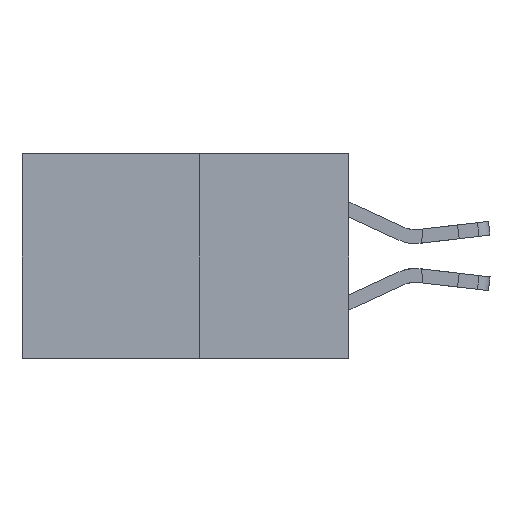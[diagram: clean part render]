
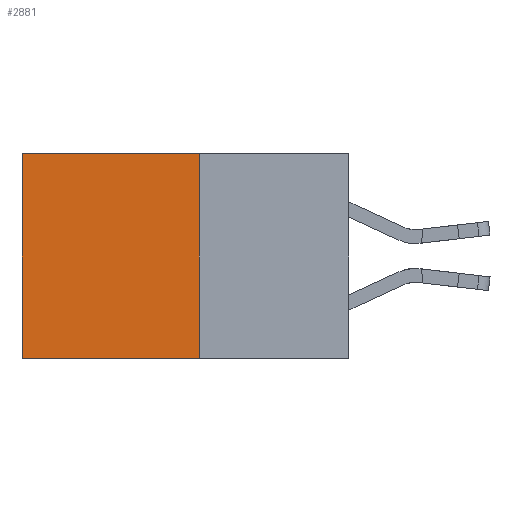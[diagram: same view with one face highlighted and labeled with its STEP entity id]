
A CAD part, left-side view. The second image highlights one B-rep face of the part: STEP entity #2881.
In plain terms, the highlighted planar face has unit normal (-1, 0, 0).
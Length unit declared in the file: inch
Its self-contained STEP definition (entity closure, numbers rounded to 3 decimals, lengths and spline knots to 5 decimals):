
#1489 = EDGE_CURVE ( 'NONE', #11108, #1979, #19267, .T. ) ;
#1666 = CARTESIAN_POINT ( 'NONE',  ( 0.277, 0.59, 0. ) ) ;
#1736 = LINE ( 'NONE', #14465, #20561 ) ;
#1979 = VERTEX_POINT ( 'NONE', #4286 ) ;
#2881 = ADVANCED_FACE ( 'NONE', ( #22049 ), #15849, .F. ) ;
#4286 = CARTESIAN_POINT ( 'NONE',  ( 0.277, 0.27, -0.37 ) ) ;
#4748 = DIRECTION ( 'NONE',  ( 1., 0., 0. ) ) ;
#5076 = VECTOR ( 'NONE', #12967, 39.37008 ) ;
#5095 = DIRECTION ( 'NONE',  ( 0., 1., 0. ) ) ;
#5452 = CARTESIAN_POINT ( 'NONE',  ( 0.277, 0.27, 0. ) ) ;
#7298 = ORIENTED_EDGE ( 'NONE', *, *, #11209, .T. ) ;
#7614 = DIRECTION ( 'NONE',  ( 0., 0., -1. ) ) ;
#10311 = EDGE_CURVE ( 'NONE', #1979, #20260, #1736, .T. ) ;
#10651 = LINE ( 'NONE', #5452, #5076 ) ;
#11108 = VERTEX_POINT ( 'NONE', #14743 ) ;
#11209 = EDGE_CURVE ( 'NONE', #18358, #20260, #15237, .T. ) ;
#12967 = DIRECTION ( 'NONE',  ( 0., 1., 0. ) ) ;
#14059 = CARTESIAN_POINT ( 'NONE',  ( 0.277, 0.59, -0.37 ) ) ;
#14068 = AXIS2_PLACEMENT_3D ( 'NONE', #21384, #4748, #17789 ) ;
#14348 = VECTOR ( 'NONE', #16652, 39.37008 ) ;
#14465 = CARTESIAN_POINT ( 'NONE',  ( 0.277, 0.27, -0.37 ) ) ;
#14743 = CARTESIAN_POINT ( 'NONE',  ( 0.277, 0.27, 0. ) ) ;
#14990 = CARTESIAN_POINT ( 'NONE',  ( 0.277, 0.59, -0.37 ) ) ;
#15237 = LINE ( 'NONE', #14990, #19570 ) ;
#15284 = CARTESIAN_POINT ( 'NONE',  ( 0.277, 0.27, -0.37 ) ) ;
#15849 = PLANE ( 'NONE',  #14068 ) ;
#16652 = DIRECTION ( 'NONE',  ( 0., 0., -1. ) ) ;
#17648 = EDGE_LOOP ( 'NONE', ( #7298, #19619, #20337, #18469 ) ) ;
#17789 = DIRECTION ( 'NONE',  ( 0., 0., -1. ) ) ;
#18358 = VERTEX_POINT ( 'NONE', #1666 ) ;
#18469 = ORIENTED_EDGE ( 'NONE', *, *, #24130, .T. ) ;
#19267 = LINE ( 'NONE', #15284, #14348 ) ;
#19570 = VECTOR ( 'NONE', #7614, 39.37008 ) ;
#19619 = ORIENTED_EDGE ( 'NONE', *, *, #10311, .F. ) ;
#20260 = VERTEX_POINT ( 'NONE', #14059 ) ;
#20337 = ORIENTED_EDGE ( 'NONE', *, *, #1489, .F. ) ;
#20561 = VECTOR ( 'NONE', #5095, 39.37008 ) ;
#21384 = CARTESIAN_POINT ( 'NONE',  ( 0.277, 0.27, -0.37 ) ) ;
#22049 = FACE_OUTER_BOUND ( 'NONE', #17648, .T. ) ;
#24130 = EDGE_CURVE ( 'NONE', #11108, #18358, #10651, .T. ) ;
